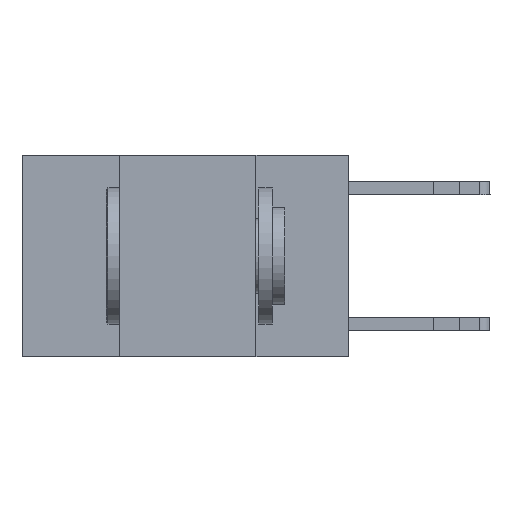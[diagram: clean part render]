
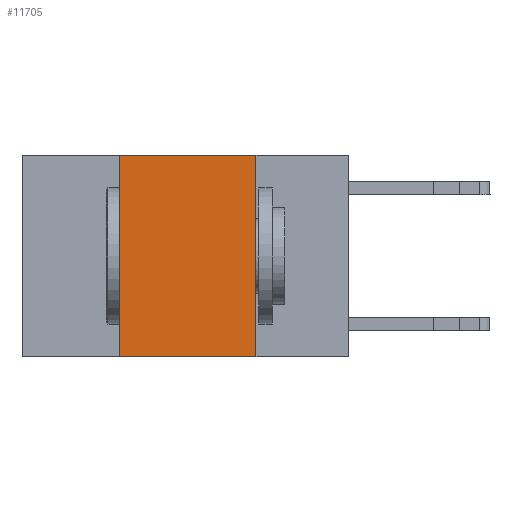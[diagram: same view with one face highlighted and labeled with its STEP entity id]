
A CAD part, left-side view. The second image highlights one B-rep face of the part: STEP entity #11705.
In plain terms, the highlighted planar face has unit normal (-1, 0, 0).
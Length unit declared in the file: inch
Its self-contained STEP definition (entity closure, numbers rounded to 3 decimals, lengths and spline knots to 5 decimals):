
#116 = DIRECTION ( 'NONE',  ( 0., -1., 0. ) ) ;
#1247 = DIRECTION ( 'NONE',  ( 0., 0., -1. ) ) ;
#1270 = CARTESIAN_POINT ( 'NONE',  ( 0., 0.6, -0.37 ) ) ;
#1383 = PLANE ( 'NONE',  #11003 ) ;
#1512 = CARTESIAN_POINT ( 'NONE',  ( 0., 0.17, 0. ) ) ;
#2874 = DIRECTION ( 'NONE',  ( 0., 0., 1. ) ) ;
#3089 = EDGE_CURVE ( 'NONE', #9679, #7723, #5610, .T. ) ;
#3527 = CARTESIAN_POINT ( 'NONE',  ( 0., 0.6, 0. ) ) ;
#4070 = DIRECTION ( 'NONE',  ( 0., 0., -1. ) ) ;
#4236 = CARTESIAN_POINT ( 'NONE',  ( 0., 0.42, 0. ) ) ;
#4580 = ORIENTED_EDGE ( 'NONE', *, *, #3089, .F. ) ;
#5110 = VECTOR ( 'NONE', #116, 39.37008 ) ;
#5486 = LINE ( 'NONE', #12253, #14143 ) ;
#5532 = CARTESIAN_POINT ( 'NONE',  ( 0., 0.6, 0. ) ) ;
#5610 = LINE ( 'NONE', #13456, #7240 ) ;
#6265 = EDGE_LOOP ( 'NONE', ( #4580, #9911, #9895, #13969 ) ) ;
#6461 = DIRECTION ( 'NONE',  ( 0., -1., 0. ) ) ;
#6842 = EDGE_CURVE ( 'NONE', #14721, #7723, #7077, .T. ) ;
#7077 = LINE ( 'NONE', #1270, #5110 ) ;
#7240 = VECTOR ( 'NONE', #4070, 39.37008 ) ;
#7723 = VERTEX_POINT ( 'NONE', #10326 ) ;
#7832 = LINE ( 'NONE', #5532, #14747 ) ;
#8195 = DIRECTION ( 'NONE',  ( 1., 0., 0. ) ) ;
#9679 = VERTEX_POINT ( 'NONE', #1512 ) ;
#9822 = EDGE_CURVE ( 'NONE', #14721, #14136, #5486, .T. ) ;
#9895 = ORIENTED_EDGE ( 'NONE', *, *, #9822, .F. ) ;
#9911 = ORIENTED_EDGE ( 'NONE', *, *, #14565, .F. ) ;
#10326 = CARTESIAN_POINT ( 'NONE',  ( 0., 0.17, -0.37 ) ) ;
#11003 = AXIS2_PLACEMENT_3D ( 'NONE', #3527, #8195, #1247 ) ;
#11285 = CARTESIAN_POINT ( 'NONE',  ( 0., 0.42, -0.37 ) ) ;
#11705 = ADVANCED_FACE ( 'NONE', ( #11836 ), #1383, .F. ) ;
#11836 = FACE_OUTER_BOUND ( 'NONE', #6265, .T. ) ;
#12253 = CARTESIAN_POINT ( 'NONE',  ( 0., 0.42, 0. ) ) ;
#13456 = CARTESIAN_POINT ( 'NONE',  ( 0., 0.17, 0. ) ) ;
#13969 = ORIENTED_EDGE ( 'NONE', *, *, #6842, .T. ) ;
#14136 = VERTEX_POINT ( 'NONE', #4236 ) ;
#14143 = VECTOR ( 'NONE', #2874, 39.37008 ) ;
#14565 = EDGE_CURVE ( 'NONE', #14136, #9679, #7832, .T. ) ;
#14721 = VERTEX_POINT ( 'NONE', #11285 ) ;
#14747 = VECTOR ( 'NONE', #6461, 39.37008 ) ;
